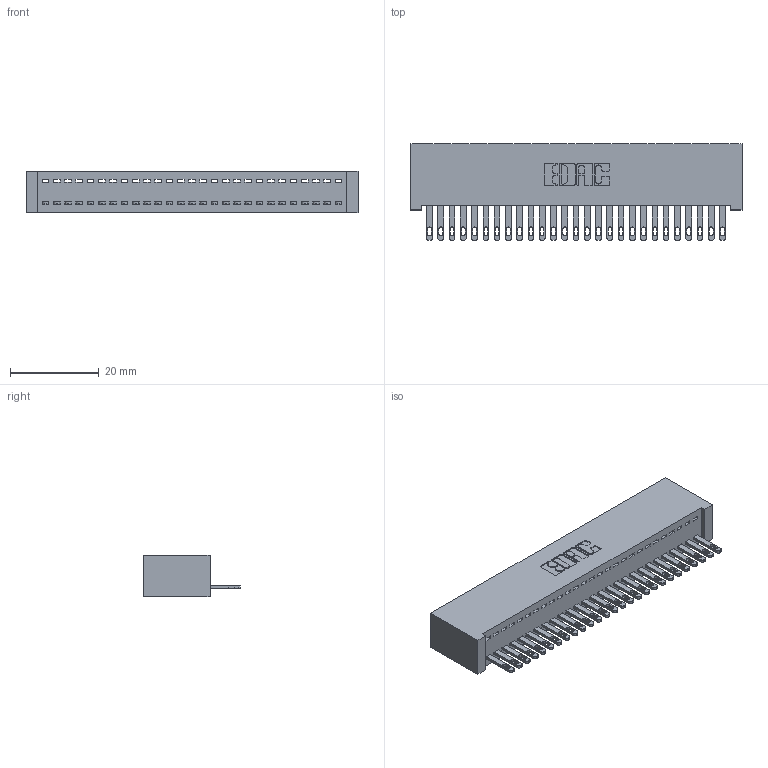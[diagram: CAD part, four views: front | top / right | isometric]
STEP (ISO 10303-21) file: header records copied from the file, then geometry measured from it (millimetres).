
FILE_DESCRIPTION (( 'STEP AP203' ), '1' );
FILE_NAME ('342-027-500-101.STEP', '2019-10-02T01:54:39', ( '' ), ( '' ), 'SwSTEP 2.0', 'SolidWorks 2016', '' );
FILE_SCHEMA (( 'CONFIG_CONTROL_DESIGN' ));
Length unit declared in the file: inch
Products named in the file (3): 345-292-001_345-293-100; 342-027-500-101; 342 Part_Lugless
Assembly tree (28 placements, depth 2):
  342-027-500-101
    342 Part_Lugless
    345-292-001_345-293-100  x27
Bounding box: 74.83 x 21.85 x 9.4 mm (x, y, z)
Volume: 6931.4 mm3; surface area: 10274.8 mm2
Topology: 28 solids, 28 shells, 1560 faces, 4811 edges, 3206 vertices
Faces by surface type: plane 1034, cylinder 526
Entity records: 17967 total; most frequent: CARTESIAN_POINT 3107, ORIENTED_EDGE 3070, DIRECTION 2645, EDGE_CURVE 1535, VECTOR 1411, LINE 1411, VERTEX_POINT 1022, AXIS2_PLACEMENT_3D 617
